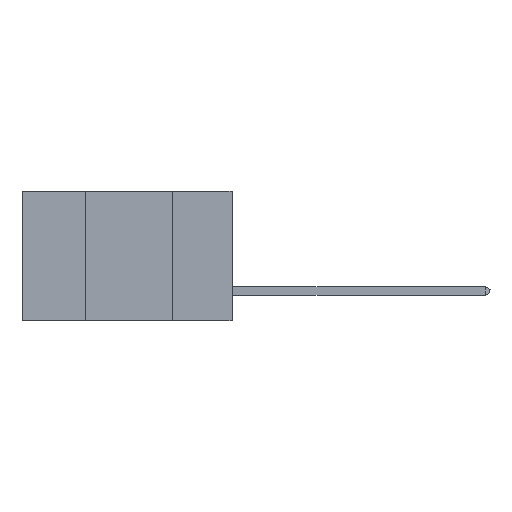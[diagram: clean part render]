
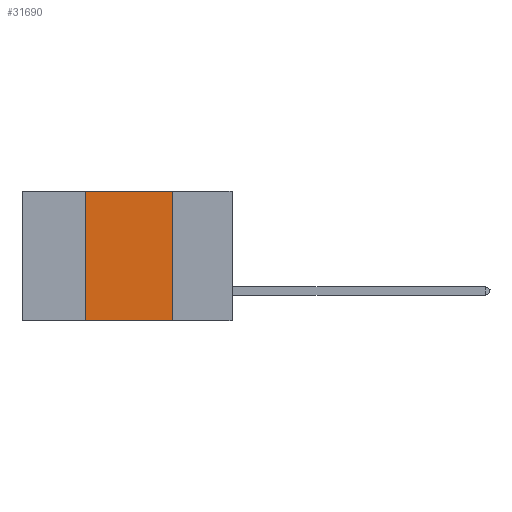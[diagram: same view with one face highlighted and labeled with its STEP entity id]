
A CAD part, left-side view. The second image highlights one B-rep face of the part: STEP entity #31690.
In plain terms, the highlighted planar face has unit normal (-1, 0, 0).
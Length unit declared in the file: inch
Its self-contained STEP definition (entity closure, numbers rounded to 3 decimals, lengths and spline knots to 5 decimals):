
#2399 = VERTEX_POINT ( 'NONE', #49302 ) ;
#3079 = VERTEX_POINT ( 'NONE', #27220 ) ;
#3698 = DIRECTION ( 'NONE',  ( 0., 0., -1. ) ) ;
#7143 = DIRECTION ( 'NONE',  ( 0., 0., -1. ) ) ;
#7542 = CARTESIAN_POINT ( 'NONE',  ( 0., 0.6, 0. ) ) ;
#7603 = VECTOR ( 'NONE', #7143, 39.37008 ) ;
#9197 = CARTESIAN_POINT ( 'NONE',  ( 0., 0.42, 0. ) ) ;
#11067 = DIRECTION ( 'NONE',  ( 0., -1., 0. ) ) ;
#11606 = DIRECTION ( 'NONE',  ( 0., -1., 0. ) ) ;
#12271 = EDGE_LOOP ( 'NONE', ( #36598, #30813, #19316, #41671 ) ) ;
#13287 = VECTOR ( 'NONE', #41688, 39.37008 ) ;
#14426 = LINE ( 'NONE', #18608, #13287 ) ;
#15160 = LINE ( 'NONE', #38526, #15742 ) ;
#15491 = CARTESIAN_POINT ( 'NONE',  ( 0., 0.17, 0. ) ) ;
#15742 = VECTOR ( 'NONE', #11606, 39.37008 ) ;
#18608 = CARTESIAN_POINT ( 'NONE',  ( 0., 0.42, 0. ) ) ;
#19316 = ORIENTED_EDGE ( 'NONE', *, *, #23033, .F. ) ;
#22487 = PLANE ( 'NONE',  #36272 ) ;
#23033 = EDGE_CURVE ( 'NONE', #3079, #39139, #14426, .T. ) ;
#26963 = EDGE_CURVE ( 'NONE', #39139, #37845, #48444, .T. ) ;
#27220 = CARTESIAN_POINT ( 'NONE',  ( 0., 0.42, -0.37 ) ) ;
#27277 = CARTESIAN_POINT ( 'NONE',  ( 0., 0.17, 0. ) ) ;
#30813 = ORIENTED_EDGE ( 'NONE', *, *, #26963, .F. ) ;
#31690 = ADVANCED_FACE ( 'NONE', ( #47546 ), #22487, .F. ) ;
#31859 = EDGE_CURVE ( 'NONE', #3079, #2399, #15160, .T. ) ;
#36272 = AXIS2_PLACEMENT_3D ( 'NONE', #41566, #41732, #3698 ) ;
#36598 = ORIENTED_EDGE ( 'NONE', *, *, #47956, .F. ) ;
#37845 = VERTEX_POINT ( 'NONE', #27277 ) ;
#38123 = LINE ( 'NONE', #15491, #7603 ) ;
#38526 = CARTESIAN_POINT ( 'NONE',  ( 0., 0.6, -0.37 ) ) ;
#39139 = VERTEX_POINT ( 'NONE', #9197 ) ;
#41263 = VECTOR ( 'NONE', #11067, 39.37008 ) ;
#41566 = CARTESIAN_POINT ( 'NONE',  ( 0., 0.6, 0. ) ) ;
#41671 = ORIENTED_EDGE ( 'NONE', *, *, #31859, .T. ) ;
#41688 = DIRECTION ( 'NONE',  ( 0., 0., 1. ) ) ;
#41732 = DIRECTION ( 'NONE',  ( 1., 0., 0. ) ) ;
#47546 = FACE_OUTER_BOUND ( 'NONE', #12271, .T. ) ;
#47956 = EDGE_CURVE ( 'NONE', #37845, #2399, #38123, .T. ) ;
#48444 = LINE ( 'NONE', #7542, #41263 ) ;
#49302 = CARTESIAN_POINT ( 'NONE',  ( 0., 0.17, -0.37 ) ) ;
